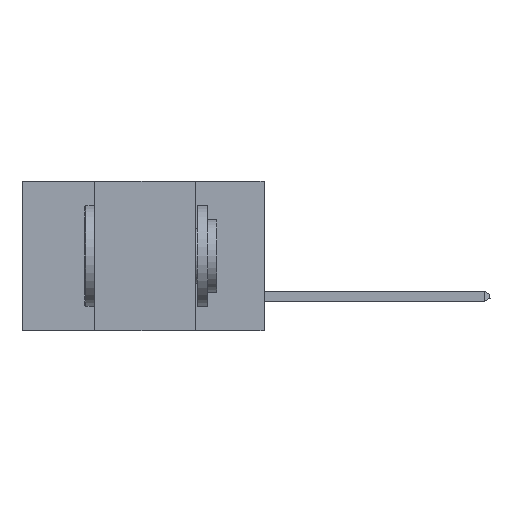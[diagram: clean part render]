
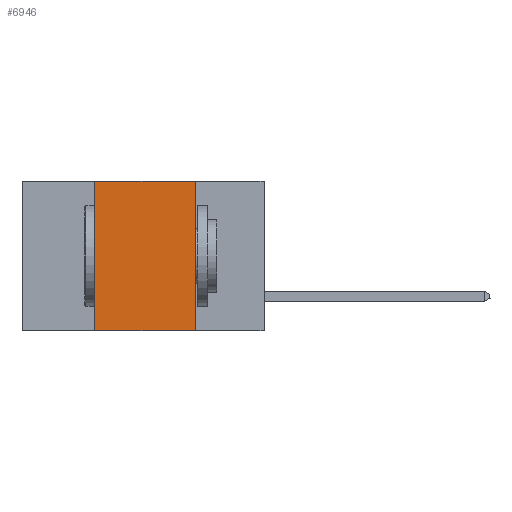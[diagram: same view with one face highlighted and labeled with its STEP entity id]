
A CAD part, left-side view. The second image highlights one B-rep face of the part: STEP entity #6946.
In plain terms, the highlighted planar face has unit normal (-1, 0, 0).
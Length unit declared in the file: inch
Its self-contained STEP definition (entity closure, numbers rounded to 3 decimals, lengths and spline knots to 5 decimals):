
#225 = VECTOR ( 'NONE', #2315, 39.37008 ) ;
#595 = DIRECTION ( 'NONE',  ( 0., 0., 1. ) ) ;
#1112 = DIRECTION ( 'NONE',  ( 0., 0., -1. ) ) ;
#2315 = DIRECTION ( 'NONE',  ( 0., 0., -1. ) ) ;
#2599 = EDGE_CURVE ( 'NONE', #5967, #10168, #14210, .T. ) ;
#3859 = CARTESIAN_POINT ( 'NONE',  ( 0., 0.17, -0.37 ) ) ;
#3875 = FACE_OUTER_BOUND ( 'NONE', #11896, .T. ) ;
#3958 = CARTESIAN_POINT ( 'NONE',  ( 0., 0.17, 0. ) ) ;
#4382 = VECTOR ( 'NONE', #10828, 39.37008 ) ;
#4978 = ORIENTED_EDGE ( 'NONE', *, *, #12846, .F. ) ;
#5505 = VERTEX_POINT ( 'NONE', #3859 ) ;
#5680 = LINE ( 'NONE', #5982, #225 ) ;
#5901 = ORIENTED_EDGE ( 'NONE', *, *, #8515, .F. ) ;
#5967 = VERTEX_POINT ( 'NONE', #12659 ) ;
#5982 = CARTESIAN_POINT ( 'NONE',  ( 0., 0.17, 0. ) ) ;
#6121 = CARTESIAN_POINT ( 'NONE',  ( 0., 0.6, 0. ) ) ;
#6168 = DIRECTION ( 'NONE',  ( 0., -1., 0. ) ) ;
#6667 = VERTEX_POINT ( 'NONE', #8513 ) ;
#6865 = EDGE_CURVE ( 'NONE', #6667, #5505, #10927, .T. ) ;
#6946 = ADVANCED_FACE ( 'NONE', ( #3875 ), #12946, .F. ) ;
#7059 = CARTESIAN_POINT ( 'NONE',  ( 0., 0.6, 0. ) ) ;
#7412 = VECTOR ( 'NONE', #6168, 39.37008 ) ;
#7774 = ORIENTED_EDGE ( 'NONE', *, *, #2599, .F. ) ;
#8259 = DIRECTION ( 'NONE',  ( 1., 0., 0. ) ) ;
#8513 = CARTESIAN_POINT ( 'NONE',  ( 0., 0.42, -0.37 ) ) ;
#8515 = EDGE_CURVE ( 'NONE', #6667, #5967, #10055, .T. ) ;
#9484 = CARTESIAN_POINT ( 'NONE',  ( 0., 0.6, -0.37 ) ) ;
#10055 = LINE ( 'NONE', #11078, #12094 ) ;
#10168 = VERTEX_POINT ( 'NONE', #3958 ) ;
#10828 = DIRECTION ( 'NONE',  ( 0., -1., 0. ) ) ;
#10927 = LINE ( 'NONE', #9484, #7412 ) ;
#11078 = CARTESIAN_POINT ( 'NONE',  ( 0., 0.42, 0. ) ) ;
#11896 = EDGE_LOOP ( 'NONE', ( #4978, #7774, #5901, #15442 ) ) ;
#12094 = VECTOR ( 'NONE', #595, 39.37008 ) ;
#12659 = CARTESIAN_POINT ( 'NONE',  ( 0., 0.42, 0. ) ) ;
#12846 = EDGE_CURVE ( 'NONE', #10168, #5505, #5680, .T. ) ;
#12946 = PLANE ( 'NONE',  #13669 ) ;
#13669 = AXIS2_PLACEMENT_3D ( 'NONE', #7059, #8259, #1112 ) ;
#14210 = LINE ( 'NONE', #6121, #4382 ) ;
#15442 = ORIENTED_EDGE ( 'NONE', *, *, #6865, .T. ) ;
